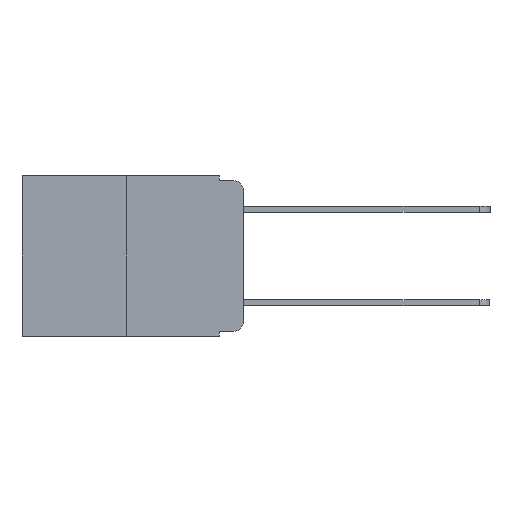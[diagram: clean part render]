
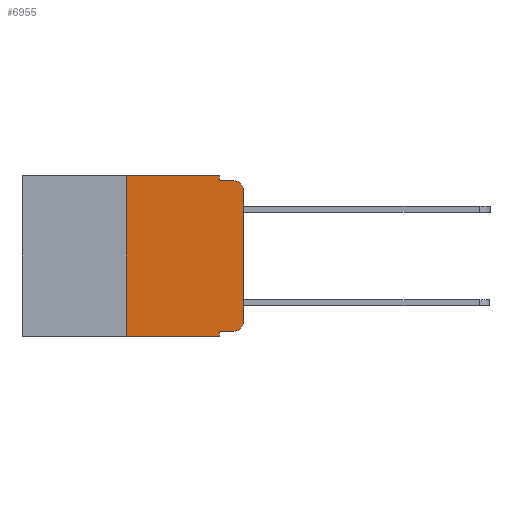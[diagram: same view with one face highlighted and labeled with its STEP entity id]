
A CAD part, left-side view. The second image highlights one B-rep face of the part: STEP entity #6955.
In plain terms, the highlighted planar face has unit normal (-1, 0, 0).
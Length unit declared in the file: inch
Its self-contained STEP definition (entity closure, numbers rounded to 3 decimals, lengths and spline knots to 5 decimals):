
#53 = EDGE_CURVE ( 'NONE', #4471, #6793, #2828, .T. ) ;
#173 = CARTESIAN_POINT ( 'NONE',  ( 0., 0.051, -0.01 ) ) ;
#349 = DIRECTION ( 'NONE',  ( 0., 0., -1. ) ) ;
#494 = EDGE_LOOP ( 'NONE', ( #9022, #9186, #9889, #10017, #15889, #10110, #15641, #1022, #1467, #2515 ) ) ;
#1022 = ORIENTED_EDGE ( 'NONE', *, *, #6798, .F. ) ;
#1467 = ORIENTED_EDGE ( 'NONE', *, *, #53, .T. ) ;
#1738 = VERTEX_POINT ( 'NONE', #19410 ) ;
#2126 = EDGE_CURVE ( 'NONE', #11198, #1738, #16526, .T. ) ;
#2515 = ORIENTED_EDGE ( 'NONE', *, *, #16880, .T. ) ;
#2828 = LINE ( 'NONE', #14954, #7667 ) ;
#2933 = CARTESIAN_POINT ( 'NONE',  ( 0., 0.02, -0.333 ) ) ;
#3083 = DIRECTION ( 'NONE',  ( 0., 0., -1. ) ) ;
#3308 = DIRECTION ( 'NONE',  ( 0., -1., 0. ) ) ;
#3419 = LINE ( 'NONE', #6242, #19494 ) ;
#4471 = VERTEX_POINT ( 'NONE', #17329 ) ;
#4523 = CARTESIAN_POINT ( 'NONE',  ( 0., 0., -0.313 ) ) ;
#4689 = FACE_OUTER_BOUND ( 'NONE', #494, .T. ) ;
#4890 = EDGE_CURVE ( 'NONE', #13785, #8093, #15033, .T. ) ;
#5495 = VECTOR ( 'NONE', #10542, 39.37008 ) ;
#5728 = DIRECTION ( 'NONE',  ( 0., -1., 0. ) ) ;
#5737 = CARTESIAN_POINT ( 'NONE',  ( 0., 0.25, 0. ) ) ;
#6242 = CARTESIAN_POINT ( 'NONE',  ( 0., 0.051, 0. ) ) ;
#6485 = VERTEX_POINT ( 'NONE', #14828 ) ;
#6731 = DIRECTION ( 'NONE',  ( 0., 0., -1. ) ) ;
#6793 = VERTEX_POINT ( 'NONE', #2933 ) ;
#6798 = EDGE_CURVE ( 'NONE', #4471, #11187, #3419, .T. ) ;
#6955 = ADVANCED_FACE ( 'NONE', ( #4689 ), #14473, .F. ) ;
#7667 = VECTOR ( 'NONE', #5728, 39.37008 ) ;
#7829 = CIRCLE ( 'NONE', #17323, 0.02 ) ;
#7836 = DIRECTION ( 'NONE',  ( 0., 0., -1. ) ) ;
#8093 = VERTEX_POINT ( 'NONE', #18081 ) ;
#8124 = DIRECTION ( 'NONE',  ( -1., 0., 0. ) ) ;
#9022 = ORIENTED_EDGE ( 'NONE', *, *, #2126, .T. ) ;
#9151 = CARTESIAN_POINT ( 'NONE',  ( 0., 0.02, -0.01 ) ) ;
#9186 = ORIENTED_EDGE ( 'NONE', *, *, #20348, .T. ) ;
#9266 = LINE ( 'NONE', #5737, #5495 ) ;
#9443 = CIRCLE ( 'NONE', #14767, 0.02 ) ;
#9575 = LINE ( 'NONE', #18843, #14138 ) ;
#9865 = CARTESIAN_POINT ( 'NONE',  ( 0., 0.473, 0. ) ) ;
#9889 = ORIENTED_EDGE ( 'NONE', *, *, #12187, .F. ) ;
#10017 = ORIENTED_EDGE ( 'NONE', *, *, #4890, .F. ) ;
#10110 = ORIENTED_EDGE ( 'NONE', *, *, #14740, .F. ) ;
#10190 = DIRECTION ( 'NONE',  ( -1., 0., 0. ) ) ;
#10542 = DIRECTION ( 'NONE',  ( 0., 0., 1. ) ) ;
#10899 = CARTESIAN_POINT ( 'NONE',  ( 0., 0.051, 0. ) ) ;
#11143 = CARTESIAN_POINT ( 'NONE',  ( 0., 0.051, 0. ) ) ;
#11187 = VERTEX_POINT ( 'NONE', #15408 ) ;
#11198 = VERTEX_POINT ( 'NONE', #4523 ) ;
#11268 = DIRECTION ( 'NONE',  ( 0., -1., 0. ) ) ;
#12187 = EDGE_CURVE ( 'NONE', #8093, #20079, #20029, .T. ) ;
#12435 = VECTOR ( 'NONE', #13046, 39.37008 ) ;
#13046 = DIRECTION ( 'NONE',  ( 0., -1., 0. ) ) ;
#13160 = EDGE_CURVE ( 'NONE', #19777, #11187, #9575, .T. ) ;
#13785 = VERTEX_POINT ( 'NONE', #10899 ) ;
#14138 = VECTOR ( 'NONE', #3308, 39.37008 ) ;
#14157 = LINE ( 'NONE', #17309, #16757 ) ;
#14473 = PLANE ( 'NONE',  #16517 ) ;
#14740 = EDGE_CURVE ( 'NONE', #19777, #6485, #9266, .T. ) ;
#14767 = AXIS2_PLACEMENT_3D ( 'NONE', #17320, #8124, #18857 ) ;
#14828 = CARTESIAN_POINT ( 'NONE',  ( 0., 0.25, 0. ) ) ;
#14954 = CARTESIAN_POINT ( 'NONE',  ( 0., 0.051, -0.333 ) ) ;
#15033 = LINE ( 'NONE', #11143, #19527 ) ;
#15408 = CARTESIAN_POINT ( 'NONE',  ( 0., 0.051, -0.343 ) ) ;
#15641 = ORIENTED_EDGE ( 'NONE', *, *, #13160, .T. ) ;
#15889 = ORIENTED_EDGE ( 'NONE', *, *, #19699, .F. ) ;
#15996 = DIRECTION ( 'NONE',  ( 1., 0., 0. ) ) ;
#16517 = AXIS2_PLACEMENT_3D ( 'NONE', #9865, #15996, #6731 ) ;
#16526 = LINE ( 'NONE', #16754, #17458 ) ;
#16754 = CARTESIAN_POINT ( 'NONE',  ( 0., 0., 0. ) ) ;
#16757 = VECTOR ( 'NONE', #11268, 39.37008 ) ;
#16880 = EDGE_CURVE ( 'NONE', #6793, #11198, #9443, .T. ) ;
#17309 = CARTESIAN_POINT ( 'NONE',  ( 0., 0.473, 0. ) ) ;
#17320 = CARTESIAN_POINT ( 'NONE',  ( 0., 0.02, -0.313 ) ) ;
#17323 = AXIS2_PLACEMENT_3D ( 'NONE', #19284, #10190, #349 ) ;
#17329 = CARTESIAN_POINT ( 'NONE',  ( 0., 0.051, -0.333 ) ) ;
#17458 = VECTOR ( 'NONE', #20296, 39.37008 ) ;
#17498 = CARTESIAN_POINT ( 'NONE',  ( 0., 0.25, -0.343 ) ) ;
#18081 = CARTESIAN_POINT ( 'NONE',  ( 0., 0.051, -0.01 ) ) ;
#18843 = CARTESIAN_POINT ( 'NONE',  ( 0., 0.473, -0.343 ) ) ;
#18857 = DIRECTION ( 'NONE',  ( 0., 0., -1. ) ) ;
#19284 = CARTESIAN_POINT ( 'NONE',  ( 0., 0.02, -0.03 ) ) ;
#19410 = CARTESIAN_POINT ( 'NONE',  ( 0., 0., -0.03 ) ) ;
#19494 = VECTOR ( 'NONE', #7836, 39.37008 ) ;
#19527 = VECTOR ( 'NONE', #3083, 39.37008 ) ;
#19699 = EDGE_CURVE ( 'NONE', #6485, #13785, #14157, .T. ) ;
#19777 = VERTEX_POINT ( 'NONE', #17498 ) ;
#20029 = LINE ( 'NONE', #173, #12435 ) ;
#20079 = VERTEX_POINT ( 'NONE', #9151 ) ;
#20296 = DIRECTION ( 'NONE',  ( 0., 0., 1. ) ) ;
#20348 = EDGE_CURVE ( 'NONE', #1738, #20079, #7829, .T. ) ;
